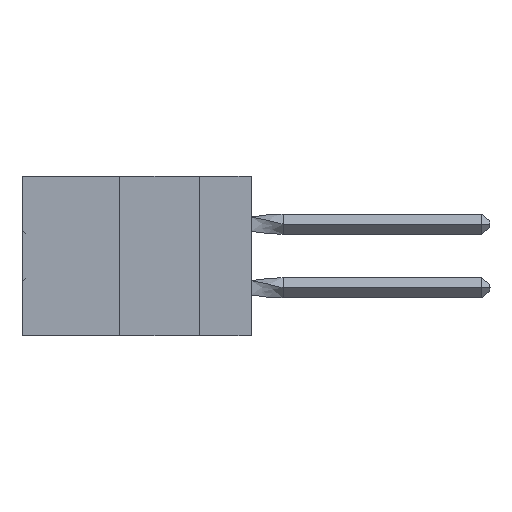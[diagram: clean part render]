
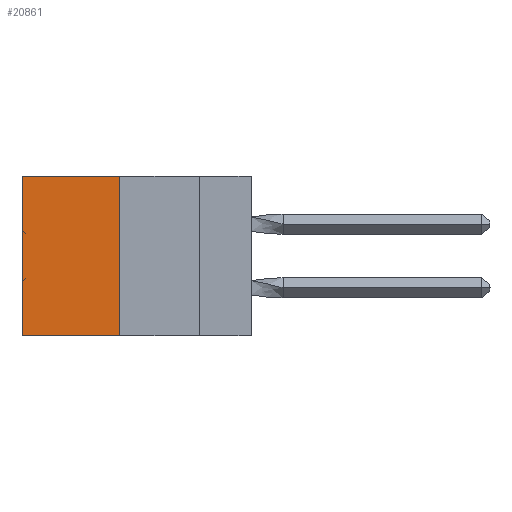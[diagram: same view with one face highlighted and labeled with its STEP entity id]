
A CAD part, left-side view. The second image highlights one B-rep face of the part: STEP entity #20861.
In plain terms, the highlighted planar face has unit normal (-1, 0, 0).
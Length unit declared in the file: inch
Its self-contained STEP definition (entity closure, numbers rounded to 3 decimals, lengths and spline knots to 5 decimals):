
#66 = EDGE_CURVE ( 'NONE', #35065, #3456, #22804, .T. ) ;
#982 = FACE_OUTER_BOUND ( 'NONE', #38205, .T. ) ;
#1225 = DIRECTION ( 'NONE',  ( 0., 1., 0. ) ) ;
#3456 = VERTEX_POINT ( 'NONE', #56153 ) ;
#9960 = DIRECTION ( 'NONE',  ( 0., 0., -1. ) ) ;
#13912 = LINE ( 'NONE', #23998, #55761 ) ;
#13992 = EDGE_CURVE ( 'NONE', #29461, #42068, #58911, .T. ) ;
#14459 = CARTESIAN_POINT ( 'NONE',  ( 0.305, 0.413, -0.5 ) ) ;
#15044 = ORIENTED_EDGE ( 'NONE', *, *, #15153, .F. ) ;
#15153 = EDGE_CURVE ( 'NONE', #42068, #3456, #19913, .T. ) ;
#16378 = ORIENTED_EDGE ( 'NONE', *, *, #13992, .F. ) ;
#17895 = VECTOR ( 'NONE', #23673, 39.37008 ) ;
#18739 = DIRECTION ( 'NONE',  ( 1., 0., 0. ) ) ;
#18950 = CARTESIAN_POINT ( 'NONE',  ( 0.305, 0.72, 0. ) ) ;
#19797 = CARTESIAN_POINT ( 'NONE',  ( 0.305, 0.413, 0. ) ) ;
#19913 = LINE ( 'NONE', #57362, #36030 ) ;
#20361 = ORIENTED_EDGE ( 'NONE', *, *, #49271, .T. ) ;
#20861 = ADVANCED_FACE ( 'NONE', ( #982 ), #56048, .F. ) ;
#22804 = LINE ( 'NONE', #37207, #36072 ) ;
#23673 = DIRECTION ( 'NONE',  ( 0., 0., -1. ) ) ;
#23998 = CARTESIAN_POINT ( 'NONE',  ( 0.305, 0.413, 0. ) ) ;
#24596 = CARTESIAN_POINT ( 'NONE',  ( 0.305, 0.413, -0.5 ) ) ;
#27554 = DIRECTION ( 'NONE',  ( 0., 0., -1. ) ) ;
#29461 = VERTEX_POINT ( 'NONE', #19797 ) ;
#35065 = VERTEX_POINT ( 'NONE', #18950 ) ;
#36030 = VECTOR ( 'NONE', #1225, 39.37008 ) ;
#36072 = VECTOR ( 'NONE', #9960, 39.37008 ) ;
#37207 = CARTESIAN_POINT ( 'NONE',  ( 0.305, 0.72, -0.5 ) ) ;
#37607 = ORIENTED_EDGE ( 'NONE', *, *, #66, .T. ) ;
#38205 = EDGE_LOOP ( 'NONE', ( #37607, #15044, #16378, #20361 ) ) ;
#42068 = VERTEX_POINT ( 'NONE', #24596 ) ;
#42131 = CARTESIAN_POINT ( 'NONE',  ( 0.305, 0.413, -0.5 ) ) ;
#43271 = DIRECTION ( 'NONE',  ( 0., 1., 0. ) ) ;
#49271 = EDGE_CURVE ( 'NONE', #29461, #35065, #13912, .T. ) ;
#55761 = VECTOR ( 'NONE', #43271, 39.37008 ) ;
#56048 = PLANE ( 'NONE',  #59199 ) ;
#56153 = CARTESIAN_POINT ( 'NONE',  ( 0.305, 0.72, -0.5 ) ) ;
#57362 = CARTESIAN_POINT ( 'NONE',  ( 0.305, 0.413, -0.5 ) ) ;
#58911 = LINE ( 'NONE', #14459, #17895 ) ;
#59199 = AXIS2_PLACEMENT_3D ( 'NONE', #42131, #18739, #27554 ) ;
